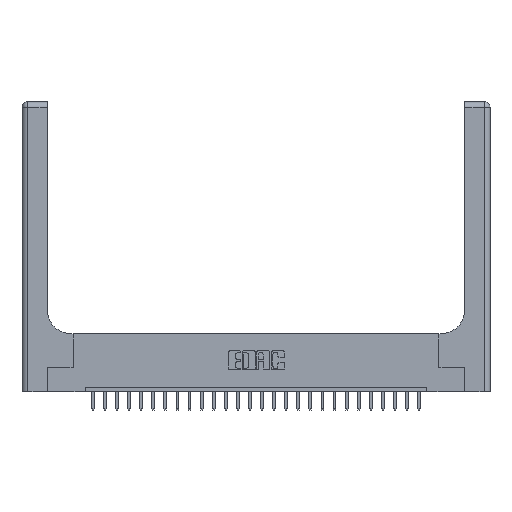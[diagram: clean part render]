
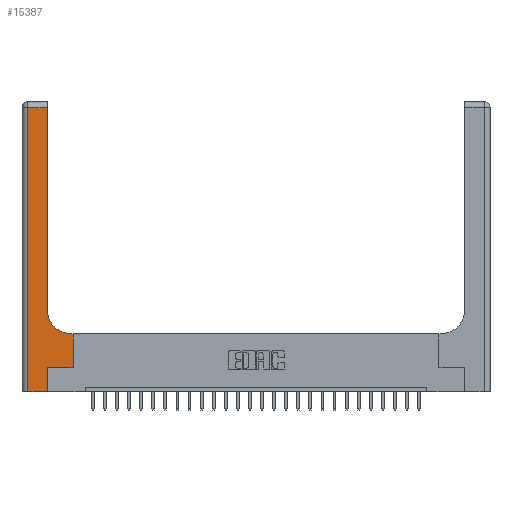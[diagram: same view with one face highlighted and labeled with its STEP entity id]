
A CAD part, top view. The second image highlights one B-rep face of the part: STEP entity #15387.
In plain terms, the highlighted planar face has unit normal (0, 0, 1).
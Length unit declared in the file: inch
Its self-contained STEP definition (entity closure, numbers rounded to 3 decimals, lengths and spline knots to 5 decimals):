
#211 = LINE ( 'NONE', #5885, #19232 ) ;
#563 = EDGE_CURVE ( 'NONE', #7178, #11018, #5090, .T. ) ;
#711 = VERTEX_POINT ( 'NONE', #1588 ) ;
#927 = DIRECTION ( 'NONE',  ( 1., 0., 0. ) ) ;
#930 = CARTESIAN_POINT ( 'NONE',  ( 0.528, 0.6, 0.37 ) ) ;
#974 = DIRECTION ( 'NONE',  ( 0., 1., 0. ) ) ;
#976 = EDGE_CURVE ( 'NONE', #21219, #7178, #211, .T. ) ;
#1000 = CARTESIAN_POINT ( 'NONE',  ( 0., 3., 0.37 ) ) ;
#1371 = EDGE_LOOP ( 'NONE', ( #14286, #14108, #17900, #22953, #22572, #3142, #17459, #21050, #18928 ) ) ;
#1588 = CARTESIAN_POINT ( 'NONE',  ( 0.26, 0.85, 0.37 ) ) ;
#2365 = LINE ( 'NONE', #4237, #23727 ) ;
#3142 = ORIENTED_EDGE ( 'NONE', *, *, #563, .T. ) ;
#4236 = DIRECTION ( 'NONE',  ( 1., 0., 0. ) ) ;
#4237 = CARTESIAN_POINT ( 'NONE',  ( 0.26, 0.6, 0.37 ) ) ;
#4404 = LINE ( 'NONE', #11020, #12794 ) ;
#4657 = CARTESIAN_POINT ( 'NONE',  ( 0.265, 0.25, 0.37 ) ) ;
#4692 = EDGE_CURVE ( 'NONE', #9582, #14350, #6514, .T. ) ;
#4734 = DIRECTION ( 'NONE',  ( 0., 0., -1. ) ) ;
#4826 = CARTESIAN_POINT ( 'NONE',  ( 0.51, 0.6, 0.37 ) ) ;
#5090 = LINE ( 'NONE', #4657, #8699 ) ;
#5345 = EDGE_CURVE ( 'NONE', #14350, #6122, #9237, .T. ) ;
#5885 = CARTESIAN_POINT ( 'NONE',  ( 0.265, 0., 0.37 ) ) ;
#5954 = CARTESIAN_POINT ( 'NONE',  ( 0.51, 0.85, 0.37 ) ) ;
#6122 = VERTEX_POINT ( 'NONE', #19207 ) ;
#6514 = LINE ( 'NONE', #17988, #10441 ) ;
#6687 = CARTESIAN_POINT ( 'NONE',  ( 0.265, 0.25, 0.37 ) ) ;
#7178 = VERTEX_POINT ( 'NONE', #6687 ) ;
#7848 = DIRECTION ( 'NONE',  ( 0., 1., 0. ) ) ;
#8487 = EDGE_CURVE ( 'NONE', #13964, #13308, #2365, .T. ) ;
#8699 = VECTOR ( 'NONE', #927, 39.37008 ) ;
#8956 = LINE ( 'NONE', #20026, #10738 ) ;
#9237 = LINE ( 'NONE', #16960, #21079 ) ;
#9406 = FACE_OUTER_BOUND ( 'NONE', #1371, .T. ) ;
#9582 = VERTEX_POINT ( 'NONE', #14246 ) ;
#10079 = CARTESIAN_POINT ( 'NONE',  ( 0.528, 0.25, 0.37 ) ) ;
#10441 = VECTOR ( 'NONE', #22612, 39.37008 ) ;
#10738 = VECTOR ( 'NONE', #974, 39.37008 ) ;
#10841 = CARTESIAN_POINT ( 'NONE',  ( 0.528, 0.25, 0.37 ) ) ;
#11018 = VERTEX_POINT ( 'NONE', #10079 ) ;
#11020 = CARTESIAN_POINT ( 'NONE',  ( 0., 0., 0.37 ) ) ;
#12794 = VECTOR ( 'NONE', #17990, 39.37008 ) ;
#13308 = VERTEX_POINT ( 'NONE', #4826 ) ;
#13964 = VERTEX_POINT ( 'NONE', #930 ) ;
#14108 = ORIENTED_EDGE ( 'NONE', *, *, #4692, .T. ) ;
#14246 = CARTESIAN_POINT ( 'NONE',  ( 0.26, 2.94, 0.37 ) ) ;
#14286 = ORIENTED_EDGE ( 'NONE', *, *, #23854, .T. ) ;
#14350 = VERTEX_POINT ( 'NONE', #18976 ) ;
#14648 = DIRECTION ( 'NONE',  ( 0., 1., 0. ) ) ;
#14700 = AXIS2_PLACEMENT_3D ( 'NONE', #1000, #4734, #22035 ) ;
#15387 = ADVANCED_FACE ( 'NONE', ( #9406 ), #20143, .F. ) ;
#16960 = CARTESIAN_POINT ( 'NONE',  ( 0.06, 3., 0.37 ) ) ;
#17038 = CIRCLE ( 'NONE', #23321, 0.25 ) ;
#17459 = ORIENTED_EDGE ( 'NONE', *, *, #22088, .T. ) ;
#17900 = ORIENTED_EDGE ( 'NONE', *, *, #5345, .T. ) ;
#17988 = CARTESIAN_POINT ( 'NONE',  ( 0., 2.94, 0.37 ) ) ;
#17990 = DIRECTION ( 'NONE',  ( 1., 0., 0. ) ) ;
#18928 = ORIENTED_EDGE ( 'NONE', *, *, #21942, .T. ) ;
#18976 = CARTESIAN_POINT ( 'NONE',  ( 0.06, 2.94, 0.37 ) ) ;
#19207 = CARTESIAN_POINT ( 'NONE',  ( 0.06, 0., 0.37 ) ) ;
#19232 = VECTOR ( 'NONE', #7848, 39.37008 ) ;
#19293 = DIRECTION ( 'NONE',  ( -1., 0., 0. ) ) ;
#19410 = VECTOR ( 'NONE', #14648, 39.37008 ) ;
#20026 = CARTESIAN_POINT ( 'NONE',  ( 0.26, 3., 0.37 ) ) ;
#20143 = PLANE ( 'NONE',  #14700 ) ;
#21050 = ORIENTED_EDGE ( 'NONE', *, *, #8487, .T. ) ;
#21079 = VECTOR ( 'NONE', #21884, 39.37008 ) ;
#21104 = DIRECTION ( 'NONE',  ( 0., 0., -1. ) ) ;
#21219 = VERTEX_POINT ( 'NONE', #23653 ) ;
#21489 = LINE ( 'NONE', #10841, #19410 ) ;
#21884 = DIRECTION ( 'NONE',  ( 0., -1., 0. ) ) ;
#21942 = EDGE_CURVE ( 'NONE', #13308, #711, #17038, .T. ) ;
#22035 = DIRECTION ( 'NONE',  ( -1., 0., 0. ) ) ;
#22088 = EDGE_CURVE ( 'NONE', #11018, #13964, #21489, .T. ) ;
#22572 = ORIENTED_EDGE ( 'NONE', *, *, #976, .T. ) ;
#22612 = DIRECTION ( 'NONE',  ( -1., 0., 0. ) ) ;
#22953 = ORIENTED_EDGE ( 'NONE', *, *, #24440, .T. ) ;
#23321 = AXIS2_PLACEMENT_3D ( 'NONE', #5954, #21104, #4236 ) ;
#23653 = CARTESIAN_POINT ( 'NONE',  ( 0.265, 0., 0.37 ) ) ;
#23727 = VECTOR ( 'NONE', #19293, 39.37008 ) ;
#23854 = EDGE_CURVE ( 'NONE', #711, #9582, #8956, .T. ) ;
#24440 = EDGE_CURVE ( 'NONE', #6122, #21219, #4404, .T. ) ;
